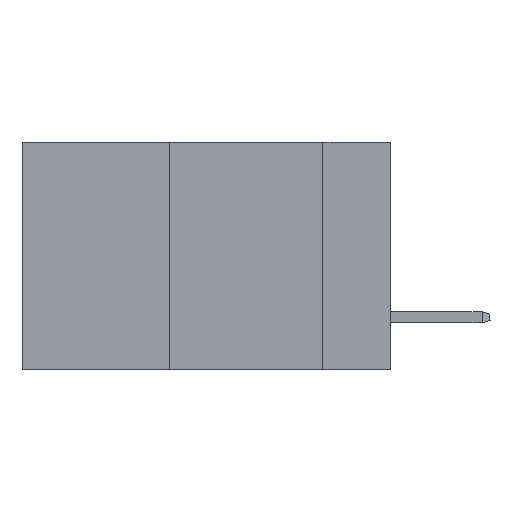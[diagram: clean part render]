
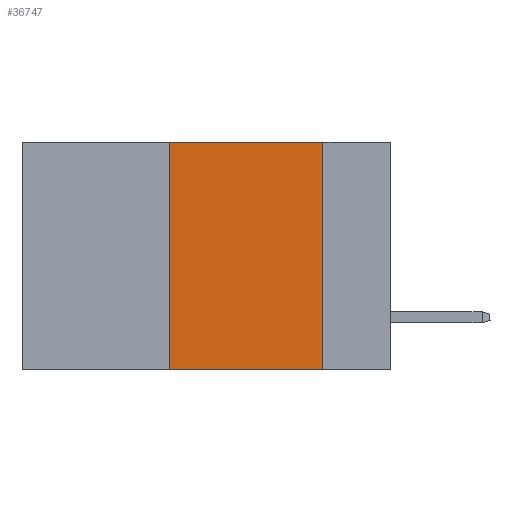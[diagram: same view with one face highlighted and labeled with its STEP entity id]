
A CAD part, left-side view. The second image highlights one B-rep face of the part: STEP entity #36747.
In plain terms, the highlighted planar face has unit normal (-1, 0, 0).
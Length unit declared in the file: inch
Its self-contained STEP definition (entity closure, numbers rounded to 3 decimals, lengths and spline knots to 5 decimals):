
#2010 = CARTESIAN_POINT ( 'NONE',  ( 0., 0.11, 0. ) ) ;
#2178 = DIRECTION ( 'NONE',  ( 0., -1., 0. ) ) ;
#3750 = CARTESIAN_POINT ( 'NONE',  ( 0., 0.11, -0.37 ) ) ;
#3770 = DIRECTION ( 'NONE',  ( 0., 0., -1. ) ) ;
#5161 = EDGE_LOOP ( 'NONE', ( #21178, #31959, #6779, #15253 ) ) ;
#5396 = DIRECTION ( 'NONE',  ( 0., 0., 1. ) ) ;
#6098 = FACE_OUTER_BOUND ( 'NONE', #5161, .T. ) ;
#6779 = ORIENTED_EDGE ( 'NONE', *, *, #36985, .F. ) ;
#8547 = LINE ( 'NONE', #30975, #11700 ) ;
#9999 = VECTOR ( 'NONE', #32765, 39.37008 ) ;
#11700 = VECTOR ( 'NONE', #2178, 39.37008 ) ;
#11731 = CARTESIAN_POINT ( 'NONE',  ( 0., 0.6, -0.37 ) ) ;
#14113 = VERTEX_POINT ( 'NONE', #2010 ) ;
#14862 = DIRECTION ( 'NONE',  ( 0., 0., -1. ) ) ;
#15253 = ORIENTED_EDGE ( 'NONE', *, *, #35549, .T. ) ;
#16412 = LINE ( 'NONE', #28493, #25394 ) ;
#16888 = AXIS2_PLACEMENT_3D ( 'NONE', #18229, #32880, #3770 ) ;
#17967 = CARTESIAN_POINT ( 'NONE',  ( 0., 0.11, 0. ) ) ;
#18229 = CARTESIAN_POINT ( 'NONE',  ( 0., 0.6, 0. ) ) ;
#18487 = LINE ( 'NONE', #11731, #9999 ) ;
#18541 = LINE ( 'NONE', #17967, #29328 ) ;
#20714 = CARTESIAN_POINT ( 'NONE',  ( 0., 0.36, -0.37 ) ) ;
#21178 = ORIENTED_EDGE ( 'NONE', *, *, #29508, .F. ) ;
#22198 = VERTEX_POINT ( 'NONE', #3750 ) ;
#25076 = EDGE_CURVE ( 'NONE', #27407, #14113, #8547, .T. ) ;
#25394 = VECTOR ( 'NONE', #5396, 39.37008 ) ;
#27407 = VERTEX_POINT ( 'NONE', #32454 ) ;
#28493 = CARTESIAN_POINT ( 'NONE',  ( 0., 0.36, 0. ) ) ;
#29328 = VECTOR ( 'NONE', #14862, 39.37008 ) ;
#29508 = EDGE_CURVE ( 'NONE', #14113, #22198, #18541, .T. ) ;
#30975 = CARTESIAN_POINT ( 'NONE',  ( 0., 0.6, 0. ) ) ;
#31959 = ORIENTED_EDGE ( 'NONE', *, *, #25076, .F. ) ;
#32454 = CARTESIAN_POINT ( 'NONE',  ( 0., 0.36, 0. ) ) ;
#32765 = DIRECTION ( 'NONE',  ( 0., -1., 0. ) ) ;
#32880 = DIRECTION ( 'NONE',  ( 1., 0., 0. ) ) ;
#34439 = VERTEX_POINT ( 'NONE', #20714 ) ;
#35549 = EDGE_CURVE ( 'NONE', #34439, #22198, #18487, .T. ) ;
#35788 = PLANE ( 'NONE',  #16888 ) ;
#36747 = ADVANCED_FACE ( 'NONE', ( #6098 ), #35788, .F. ) ;
#36985 = EDGE_CURVE ( 'NONE', #34439, #27407, #16412, .T. ) ;
